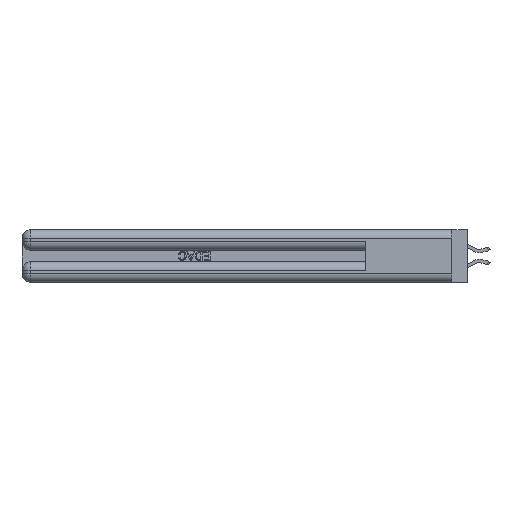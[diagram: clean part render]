
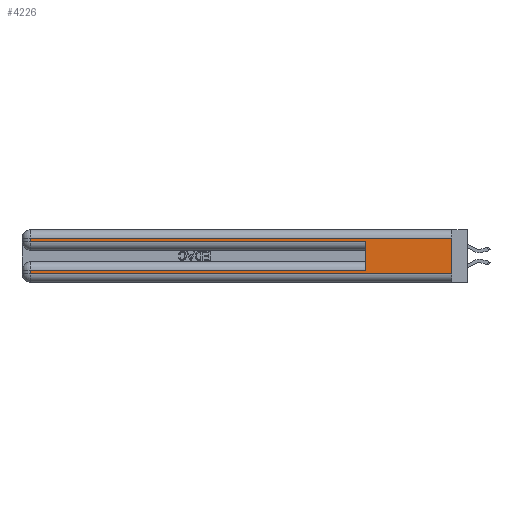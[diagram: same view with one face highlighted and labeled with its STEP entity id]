
A CAD part, left-side view. The second image highlights one B-rep face of the part: STEP entity #4226.
In plain terms, the highlighted planar face has unit normal (-1, 0, 0).
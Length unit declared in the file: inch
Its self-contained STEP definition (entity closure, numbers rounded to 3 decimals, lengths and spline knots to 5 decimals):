
#174 = VERTEX_POINT ( 'NONE', #37838 ) ;
#699 = VECTOR ( 'NONE', #12655, 39.37008 ) ;
#751 = CARTESIAN_POINT ( 'NONE',  ( 0., 2.94, 0.31 ) ) ;
#1061 = EDGE_CURVE ( 'NONE', #3852, #30396, #31021, .T. ) ;
#1409 = ORIENTED_EDGE ( 'NONE', *, *, #24496, .T. ) ;
#2197 = EDGE_CURVE ( 'NONE', #17953, #30442, #14273, .T. ) ;
#2917 = VECTOR ( 'NONE', #6745, 39.37008 ) ;
#2985 = VECTOR ( 'NONE', #11417, 39.37008 ) ;
#3368 = DIRECTION ( 'NONE',  ( 0., -1., 0. ) ) ;
#3601 = EDGE_CURVE ( 'NONE', #11041, #7965, #29469, .T. ) ;
#3628 = LINE ( 'NONE', #4143, #37141 ) ;
#3852 = VERTEX_POINT ( 'NONE', #7004 ) ;
#4072 = EDGE_LOOP ( 'NONE', ( #6463, #1409, #16744, #28632, #23921, #35618, #28630, #5044 ) ) ;
#4143 = CARTESIAN_POINT ( 'NONE',  ( 0., 0., 0.085 ) ) ;
#4226 = ADVANCED_FACE ( 'NONE', ( #8957 ), #6387, .F. ) ;
#5044 = ORIENTED_EDGE ( 'NONE', *, *, #19316, .T. ) ;
#6387 = PLANE ( 'NONE',  #37296 ) ;
#6463 = ORIENTED_EDGE ( 'NONE', *, *, #17760, .F. ) ;
#6745 = DIRECTION ( 'NONE',  ( 0., -1., 0. ) ) ;
#7004 = CARTESIAN_POINT ( 'NONE',  ( 0., 0.6, 0.085 ) ) ;
#7965 = VERTEX_POINT ( 'NONE', #10253 ) ;
#8957 = FACE_OUTER_BOUND ( 'NONE', #4072, .T. ) ;
#9223 = CARTESIAN_POINT ( 'NONE',  ( 0., 0., 0.37 ) ) ;
#10253 = CARTESIAN_POINT ( 'NONE',  ( 0., 2.94, 0.285 ) ) ;
#10809 = LINE ( 'NONE', #32367, #2917 ) ;
#10956 = DIRECTION ( 'NONE',  ( 0., 0., -1. ) ) ;
#11041 = VERTEX_POINT ( 'NONE', #751 ) ;
#11417 = DIRECTION ( 'NONE',  ( 0., 1., 0. ) ) ;
#11763 = DIRECTION ( 'NONE',  ( 0., 0., 1. ) ) ;
#12655 = DIRECTION ( 'NONE',  ( 0., 0., -1. ) ) ;
#14273 = LINE ( 'NONE', #24511, #699 ) ;
#16744 = ORIENTED_EDGE ( 'NONE', *, *, #3601, .T. ) ;
#16748 = DIRECTION ( 'NONE',  ( 0., 0., -1. ) ) ;
#16811 = VERTEX_POINT ( 'NONE', #19610 ) ;
#17760 = EDGE_CURVE ( 'NONE', #174, #16811, #33706, .T. ) ;
#17953 = VERTEX_POINT ( 'NONE', #35214 ) ;
#19316 = EDGE_CURVE ( 'NONE', #30442, #16811, #10809, .T. ) ;
#19610 = CARTESIAN_POINT ( 'NONE',  ( 0., 0., 0.06 ) ) ;
#19947 = EDGE_CURVE ( 'NONE', #7965, #30396, #36399, .T. ) ;
#20890 = CARTESIAN_POINT ( 'NONE',  ( 0., 0.6, 0.145 ) ) ;
#22137 = DIRECTION ( 'NONE',  ( 0., 1., 0. ) ) ;
#22993 = VECTOR ( 'NONE', #3368, 39.37008 ) ;
#23218 = VECTOR ( 'NONE', #11763, 39.37008 ) ;
#23921 = ORIENTED_EDGE ( 'NONE', *, *, #1061, .F. ) ;
#24118 = CARTESIAN_POINT ( 'NONE',  ( 0., 0., 0.285 ) ) ;
#24496 = EDGE_CURVE ( 'NONE', #174, #11041, #28095, .T. ) ;
#24511 = CARTESIAN_POINT ( 'NONE',  ( 0., 2.94, 0.37 ) ) ;
#25595 = CARTESIAN_POINT ( 'NONE',  ( 0., 2.94, 0.37 ) ) ;
#26577 = CARTESIAN_POINT ( 'NONE',  ( 0., 0.6, 0.285 ) ) ;
#27205 = DIRECTION ( 'NONE',  ( 1., 0., 0. ) ) ;
#28095 = LINE ( 'NONE', #29191, #2985 ) ;
#28630 = ORIENTED_EDGE ( 'NONE', *, *, #2197, .T. ) ;
#28632 = ORIENTED_EDGE ( 'NONE', *, *, #19947, .T. ) ;
#28771 = CARTESIAN_POINT ( 'NONE',  ( 0., 0., 0.37 ) ) ;
#29191 = CARTESIAN_POINT ( 'NONE',  ( 0., 0., 0.31 ) ) ;
#29469 = LINE ( 'NONE', #25595, #34126 ) ;
#30158 = DIRECTION ( 'NONE',  ( 0., 0., -1. ) ) ;
#30396 = VERTEX_POINT ( 'NONE', #26577 ) ;
#30442 = VERTEX_POINT ( 'NONE', #38145 ) ;
#31021 = LINE ( 'NONE', #20890, #23218 ) ;
#32367 = CARTESIAN_POINT ( 'NONE',  ( 0., 0., 0.06 ) ) ;
#33226 = EDGE_CURVE ( 'NONE', #3852, #17953, #3628, .T. ) ;
#33706 = LINE ( 'NONE', #28771, #36955 ) ;
#34126 = VECTOR ( 'NONE', #16748, 39.37008 ) ;
#35214 = CARTESIAN_POINT ( 'NONE',  ( 0., 2.94, 0.085 ) ) ;
#35618 = ORIENTED_EDGE ( 'NONE', *, *, #33226, .T. ) ;
#36399 = LINE ( 'NONE', #24118, #22993 ) ;
#36955 = VECTOR ( 'NONE', #10956, 39.37008 ) ;
#37141 = VECTOR ( 'NONE', #22137, 39.37008 ) ;
#37296 = AXIS2_PLACEMENT_3D ( 'NONE', #9223, #27205, #30158 ) ;
#37838 = CARTESIAN_POINT ( 'NONE',  ( 0., 0., 0.31 ) ) ;
#38145 = CARTESIAN_POINT ( 'NONE',  ( 0., 2.94, 0.06 ) ) ;
